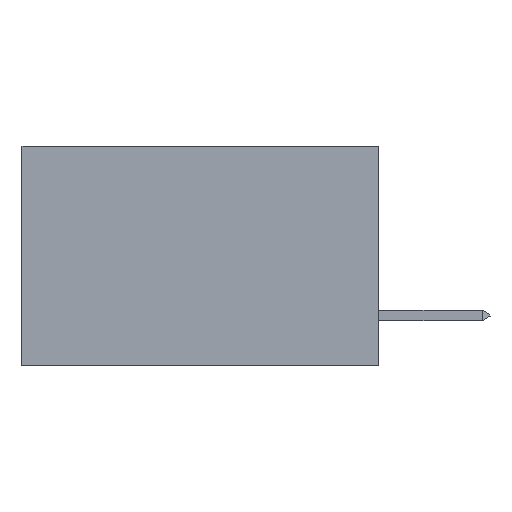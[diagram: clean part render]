
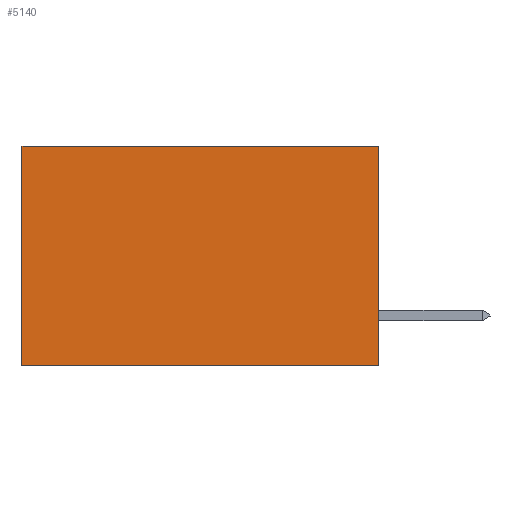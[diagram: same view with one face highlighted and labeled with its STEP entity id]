
A CAD part, left-side view. The second image highlights one B-rep face of the part: STEP entity #5140.
In plain terms, the highlighted planar face has unit normal (-1, 0, 0).
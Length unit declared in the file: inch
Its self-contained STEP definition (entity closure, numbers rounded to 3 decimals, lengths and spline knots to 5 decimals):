
#4 = VERTEX_POINT ( 'NONE', #12712 ) ;
#142 = FACE_OUTER_BOUND ( 'NONE', #12531, .T. ) ;
#513 = EDGE_CURVE ( 'NONE', #4, #7006, #10966, .T. ) ;
#522 = DIRECTION ( 'NONE',  ( 0., 1., 0. ) ) ;
#1344 = DIRECTION ( 'NONE',  ( 0., 1., 0. ) ) ;
#2615 = CARTESIAN_POINT ( 'NONE',  ( 0.298, 0., -0.37 ) ) ;
#3444 = ORIENTED_EDGE ( 'NONE', *, *, #513, .T. ) ;
#3559 = DIRECTION ( 'NONE',  ( 1., 0., 0. ) ) ;
#3735 = VERTEX_POINT ( 'NONE', #2615 ) ;
#3936 = EDGE_CURVE ( 'NONE', #6005, #3735, #9675, .T. ) ;
#4360 = ORIENTED_EDGE ( 'NONE', *, *, #12919, .T. ) ;
#4762 = DIRECTION ( 'NONE',  ( 0., 0., -1. ) ) ;
#4873 = CARTESIAN_POINT ( 'NONE',  ( 0.298, 0.6, -0.37 ) ) ;
#5036 = ORIENTED_EDGE ( 'NONE', *, *, #7547, .F. ) ;
#5076 = ORIENTED_EDGE ( 'NONE', *, *, #3936, .F. ) ;
#5140 = ADVANCED_FACE ( 'NONE', ( #142 ), #12167, .F. ) ;
#6005 = VERTEX_POINT ( 'NONE', #11299 ) ;
#6123 = LINE ( 'NONE', #11183, #11168 ) ;
#6177 = VECTOR ( 'NONE', #1344, 39.37008 ) ;
#6806 = CARTESIAN_POINT ( 'NONE',  ( 0.298, 0., 0. ) ) ;
#6904 = DIRECTION ( 'NONE',  ( 0., 0., -1. ) ) ;
#7006 = VERTEX_POINT ( 'NONE', #4873 ) ;
#7547 = EDGE_CURVE ( 'NONE', #3735, #7006, #6123, .T. ) ;
#7825 = VECTOR ( 'NONE', #13212, 39.37008 ) ;
#9016 = CARTESIAN_POINT ( 'NONE',  ( 0.298, 0.6, 0. ) ) ;
#9037 = LINE ( 'NONE', #13195, #6177 ) ;
#9675 = LINE ( 'NONE', #11940, #7825 ) ;
#10933 = AXIS2_PLACEMENT_3D ( 'NONE', #6806, #3559, #4762 ) ;
#10966 = LINE ( 'NONE', #9016, #12459 ) ;
#11168 = VECTOR ( 'NONE', #522, 39.37008 ) ;
#11183 = CARTESIAN_POINT ( 'NONE',  ( 0.298, 0., -0.37 ) ) ;
#11299 = CARTESIAN_POINT ( 'NONE',  ( 0.298, 0., 0. ) ) ;
#11940 = CARTESIAN_POINT ( 'NONE',  ( 0.298, 0., 0. ) ) ;
#12167 = PLANE ( 'NONE',  #10933 ) ;
#12459 = VECTOR ( 'NONE', #6904, 39.37008 ) ;
#12531 = EDGE_LOOP ( 'NONE', ( #3444, #5036, #5076, #4360 ) ) ;
#12712 = CARTESIAN_POINT ( 'NONE',  ( 0.298, 0.6, 0. ) ) ;
#12919 = EDGE_CURVE ( 'NONE', #6005, #4, #9037, .T. ) ;
#13195 = CARTESIAN_POINT ( 'NONE',  ( 0.298, 0., 0. ) ) ;
#13212 = DIRECTION ( 'NONE',  ( 0., 0., -1. ) ) ;
